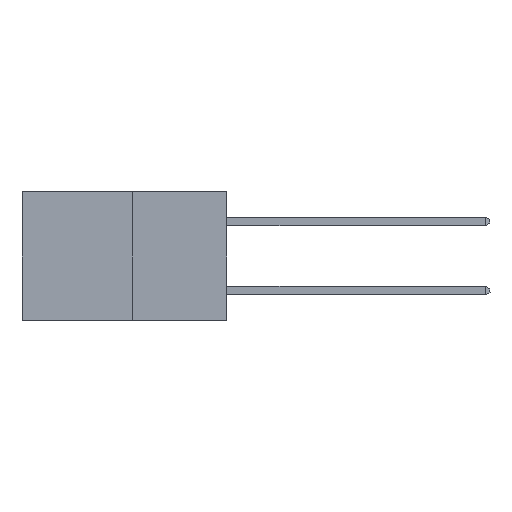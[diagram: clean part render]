
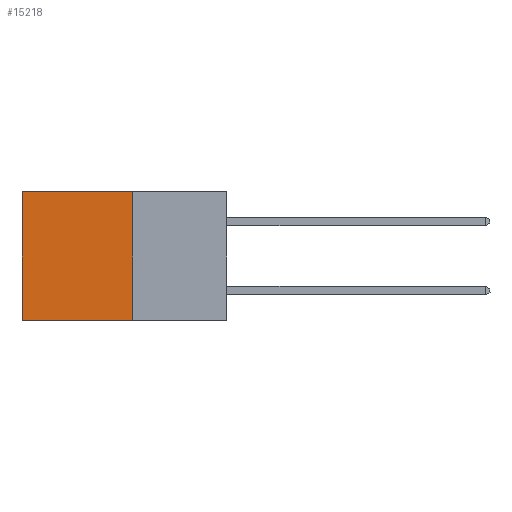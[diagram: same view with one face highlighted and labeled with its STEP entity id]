
A CAD part, left-side view. The second image highlights one B-rep face of the part: STEP entity #15218.
In plain terms, the highlighted planar face has unit normal (-1, 0, 0).
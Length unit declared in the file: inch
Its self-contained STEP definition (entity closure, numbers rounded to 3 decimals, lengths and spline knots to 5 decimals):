
#676 = FACE_OUTER_BOUND ( 'NONE', #15059, .T. ) ;
#1765 = ORIENTED_EDGE ( 'NONE', *, *, #13648, .F. ) ;
#1961 = AXIS2_PLACEMENT_3D ( 'NONE', #3312, #4989, #16852 ) ;
#2731 = CARTESIAN_POINT ( 'NONE',  ( 0.277, 0.59, -0.37 ) ) ;
#2900 = VERTEX_POINT ( 'NONE', #6969 ) ;
#3312 = CARTESIAN_POINT ( 'NONE',  ( 0.277, 0.27, -0.37 ) ) ;
#3955 = LINE ( 'NONE', #2731, #16943 ) ;
#4463 = EDGE_CURVE ( 'NONE', #20854, #10084, #18794, .T. ) ;
#4467 = CARTESIAN_POINT ( 'NONE',  ( 0.277, 0.27, -0.37 ) ) ;
#4602 = LINE ( 'NONE', #20109, #13091 ) ;
#4879 = EDGE_CURVE ( 'NONE', #20854, #5242, #13446, .T. ) ;
#4989 = DIRECTION ( 'NONE',  ( 1., 0., 0. ) ) ;
#5242 = VERTEX_POINT ( 'NONE', #4467 ) ;
#5627 = CARTESIAN_POINT ( 'NONE',  ( 0.277, 0.59, 0. ) ) ;
#6020 = ORIENTED_EDGE ( 'NONE', *, *, #17086, .T. ) ;
#6969 = CARTESIAN_POINT ( 'NONE',  ( 0.277, 0.59, -0.37 ) ) ;
#7044 = DIRECTION ( 'NONE',  ( 0., 0., -1. ) ) ;
#7764 = CARTESIAN_POINT ( 'NONE',  ( 0.277, 0.27, -0.37 ) ) ;
#8362 = VECTOR ( 'NONE', #7044, 39.37008 ) ;
#8649 = ORIENTED_EDGE ( 'NONE', *, *, #4879, .F. ) ;
#10084 = VERTEX_POINT ( 'NONE', #5627 ) ;
#10364 = CARTESIAN_POINT ( 'NONE',  ( 0.277, 0.27, 0. ) ) ;
#10571 = CARTESIAN_POINT ( 'NONE',  ( 0.277, 0.27, 0. ) ) ;
#10591 = DIRECTION ( 'NONE',  ( 0., 1., 0. ) ) ;
#11230 = DIRECTION ( 'NONE',  ( 0., 0., -1. ) ) ;
#13091 = VECTOR ( 'NONE', #20871, 39.37008 ) ;
#13446 = LINE ( 'NONE', #7764, #8362 ) ;
#13468 = PLANE ( 'NONE',  #1961 ) ;
#13648 = EDGE_CURVE ( 'NONE', #5242, #2900, #4602, .T. ) ;
#14330 = VECTOR ( 'NONE', #10591, 39.37008 ) ;
#15059 = EDGE_LOOP ( 'NONE', ( #6020, #1765, #8649, #15132 ) ) ;
#15132 = ORIENTED_EDGE ( 'NONE', *, *, #4463, .T. ) ;
#15218 = ADVANCED_FACE ( 'NONE', ( #676 ), #13468, .F. ) ;
#16852 = DIRECTION ( 'NONE',  ( 0., 0., -1. ) ) ;
#16943 = VECTOR ( 'NONE', #11230, 39.37008 ) ;
#17086 = EDGE_CURVE ( 'NONE', #10084, #2900, #3955, .T. ) ;
#18794 = LINE ( 'NONE', #10364, #14330 ) ;
#20109 = CARTESIAN_POINT ( 'NONE',  ( 0.277, 0.27, -0.37 ) ) ;
#20854 = VERTEX_POINT ( 'NONE', #10571 ) ;
#20871 = DIRECTION ( 'NONE',  ( 0., 1., 0. ) ) ;
